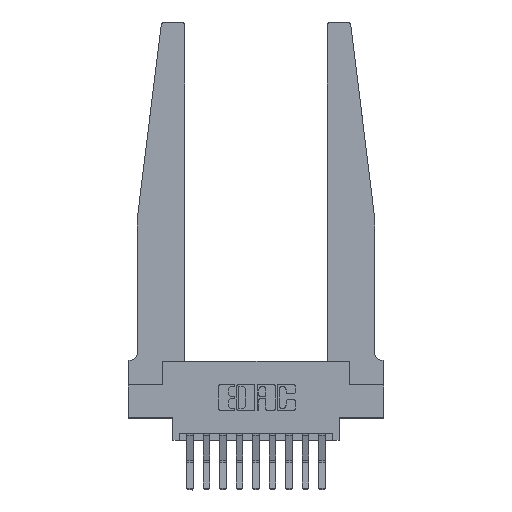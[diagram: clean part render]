
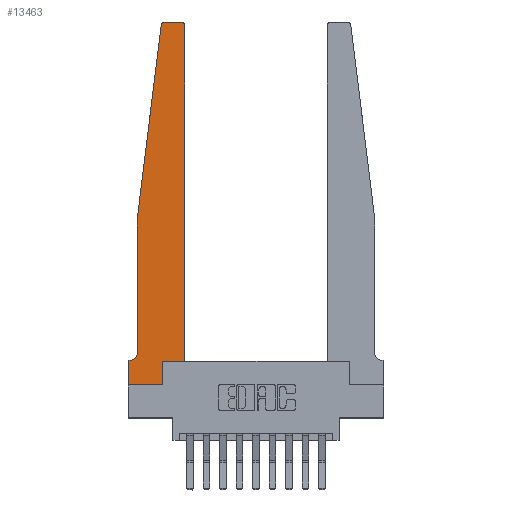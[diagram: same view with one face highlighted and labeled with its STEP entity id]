
A CAD part, top view. The second image highlights one B-rep face of the part: STEP entity #13463.
In plain terms, the highlighted planar face has unit normal (0, 0, 1).
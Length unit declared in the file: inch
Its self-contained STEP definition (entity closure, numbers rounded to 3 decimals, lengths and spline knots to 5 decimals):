
#108 = AXIS2_PLACEMENT_3D ( 'NONE', #7284, #8476, #1395 ) ;
#191 = ORIENTED_EDGE ( 'NONE', *, *, #7530, .T. ) ;
#193 = CARTESIAN_POINT ( 'NONE',  ( 0.2605, 0., 0.37 ) ) ;
#221 = VERTEX_POINT ( 'NONE', #193 ) ;
#870 = EDGE_CURVE ( 'NONE', #2707, #9263, #13168, .T. ) ;
#991 = VECTOR ( 'NONE', #13193, 39.37008 ) ;
#1066 = CARTESIAN_POINT ( 'NONE',  ( 0.395, 2.75, 0.37 ) ) ;
#1073 = LINE ( 'NONE', #15051, #13970 ) ;
#1248 = CARTESIAN_POINT ( 'NONE',  ( 0.2605, 0.18, 0.37 ) ) ;
#1303 = VERTEX_POINT ( 'NONE', #1066 ) ;
#1309 = EDGE_CURVE ( 'NONE', #4914, #3187, #11144, .T. ) ;
#1395 = DIRECTION ( 'NONE',  ( 1., 0., 0. ) ) ;
#1493 = CARTESIAN_POINT ( 'NONE',  ( 0.425, 0.18, 0.37 ) ) ;
#1557 = EDGE_CURVE ( 'NONE', #15088, #3222, #2284, .T. ) ;
#1620 = EDGE_CURVE ( 'NONE', #221, #3183, #10572, .T. ) ;
#1846 = DIRECTION ( 'NONE',  ( 1., 0., 0. ) ) ;
#2101 = CARTESIAN_POINT ( 'NONE',  ( 0., 0.1875, 0.37 ) ) ;
#2284 = LINE ( 'NONE', #1493, #11316 ) ;
#2380 = DIRECTION ( 'NONE',  ( 0., 0., 1. ) ) ;
#2623 = LINE ( 'NONE', #3178, #14767 ) ;
#2625 = VERTEX_POINT ( 'NONE', #4677 ) ;
#2666 = EDGE_CURVE ( 'NONE', #4063, #11071, #14952, .T. ) ;
#2689 = DIRECTION ( 'NONE',  ( 0., 1., 0. ) ) ;
#2707 = VERTEX_POINT ( 'NONE', #9500 ) ;
#2917 = EDGE_CURVE ( 'NONE', #3187, #4063, #2623, .T. ) ;
#3178 = CARTESIAN_POINT ( 'NONE',  ( 0.065, 0.1875, 0.37 ) ) ;
#3183 = VERTEX_POINT ( 'NONE', #1248 ) ;
#3187 = VERTEX_POINT ( 'NONE', #4842 ) ;
#3222 = VERTEX_POINT ( 'NONE', #7240 ) ;
#3589 = EDGE_CURVE ( 'NONE', #2625, #2707, #13636, .T. ) ;
#3675 = CARTESIAN_POINT ( 'NONE',  ( 0.065, 0.2375, 0.37 ) ) ;
#3740 = ORIENTED_EDGE ( 'NONE', *, *, #9920, .T. ) ;
#3920 = VECTOR ( 'NONE', #14111, 39.37008 ) ;
#4030 = CARTESIAN_POINT ( 'NONE',  ( 0.425, 0.18, 0.37 ) ) ;
#4063 = VERTEX_POINT ( 'NONE', #2101 ) ;
#4285 = ORIENTED_EDGE ( 'NONE', *, *, #3589, .T. ) ;
#4318 = VECTOR ( 'NONE', #8672, 39.37008 ) ;
#4478 = VECTOR ( 'NONE', #1846, 39.37008 ) ;
#4657 = CARTESIAN_POINT ( 'NONE',  ( 0.015, 0.2375, 0.37 ) ) ;
#4659 = EDGE_CURVE ( 'NONE', #1303, #2625, #1073, .T. ) ;
#4677 = CARTESIAN_POINT ( 'NONE',  ( 0.27653, 2.75, 0.37 ) ) ;
#4711 = DIRECTION ( 'NONE',  ( 0., 0., 1. ) ) ;
#4842 = CARTESIAN_POINT ( 'NONE',  ( 0.015, 0.1875, 0.37 ) ) ;
#4914 = VERTEX_POINT ( 'NONE', #3675 ) ;
#5268 = DIRECTION ( 'NONE',  ( 0., -1., 0. ) ) ;
#5409 = ORIENTED_EDGE ( 'NONE', *, *, #1557, .T. ) ;
#5853 = DIRECTION ( 'NONE',  ( -1., 0., 0. ) ) ;
#6107 = PLANE ( 'NONE',  #108 ) ;
#6480 = CIRCLE ( 'NONE', #12858, 0.03 ) ;
#6740 = DIRECTION ( 'NONE',  ( -1., 0., 0. ) ) ;
#6756 = EDGE_CURVE ( 'NONE', #3183, #15088, #8065, .T. ) ;
#7082 = CARTESIAN_POINT ( 'NONE',  ( 0., 0., 0.37 ) ) ;
#7240 = CARTESIAN_POINT ( 'NONE',  ( 0.425, 2.72, 0.37 ) ) ;
#7284 = CARTESIAN_POINT ( 'NONE',  ( 0., 0.1875, 0.37 ) ) ;
#7308 = CARTESIAN_POINT ( 'NONE',  ( 0., 0., 0.37 ) ) ;
#7530 = EDGE_CURVE ( 'NONE', #11071, #221, #8351, .T. ) ;
#7549 = DIRECTION ( 'NONE',  ( 1., 0., 0. ) ) ;
#7796 = ORIENTED_EDGE ( 'NONE', *, *, #14000, .T. ) ;
#8016 = DIRECTION ( 'NONE',  ( -1., 0., 0. ) ) ;
#8065 = LINE ( 'NONE', #13390, #13930 ) ;
#8351 = LINE ( 'NONE', #12380, #4478 ) ;
#8476 = DIRECTION ( 'NONE',  ( 0., 0., 1. ) ) ;
#8583 = CARTESIAN_POINT ( 'NONE',  ( 0.065, 1.25, 0.37 ) ) ;
#8672 = DIRECTION ( 'NONE',  ( 0., 1., 0. ) ) ;
#8943 = CARTESIAN_POINT ( 'NONE',  ( 0.065, 1.25, 0.37 ) ) ;
#9263 = VERTEX_POINT ( 'NONE', #8943 ) ;
#9265 = ORIENTED_EDGE ( 'NONE', *, *, #870, .T. ) ;
#9418 = CARTESIAN_POINT ( 'NONE',  ( 0.395, 2.72, 0.37 ) ) ;
#9457 = ORIENTED_EDGE ( 'NONE', *, *, #4659, .T. ) ;
#9500 = CARTESIAN_POINT ( 'NONE',  ( 0.24675, 2.72367, 0.37 ) ) ;
#9920 = EDGE_CURVE ( 'NONE', #3222, #1303, #6480, .T. ) ;
#10572 = LINE ( 'NONE', #14509, #4318 ) ;
#10616 = DIRECTION ( 'NONE',  ( 1., 0., 0. ) ) ;
#10920 = ORIENTED_EDGE ( 'NONE', *, *, #1309, .T. ) ;
#11071 = VERTEX_POINT ( 'NONE', #7308 ) ;
#11144 = CIRCLE ( 'NONE', #11884, 0.05 ) ;
#11279 = ORIENTED_EDGE ( 'NONE', *, *, #2666, .T. ) ;
#11301 = VECTOR ( 'NONE', #5268, 39.37008 ) ;
#11316 = VECTOR ( 'NONE', #2689, 39.37008 ) ;
#11429 = EDGE_LOOP ( 'NONE', ( #9457, #4285, #9265, #7796, #10920, #12386, #11279, #191, #14391, #12753, #5409, #3740 ) ) ;
#11738 = CARTESIAN_POINT ( 'NONE',  ( 0.27653, 2.72, 0.37 ) ) ;
#11884 = AXIS2_PLACEMENT_3D ( 'NONE', #4657, #12871, #5853 ) ;
#12230 = CARTESIAN_POINT ( 'NONE',  ( 0.065, 1.25, 0.37 ) ) ;
#12380 = CARTESIAN_POINT ( 'NONE',  ( 0., 0., 0.37 ) ) ;
#12386 = ORIENTED_EDGE ( 'NONE', *, *, #2917, .T. ) ;
#12405 = FACE_OUTER_BOUND ( 'NONE', #11429, .T. ) ;
#12753 = ORIENTED_EDGE ( 'NONE', *, *, #6756, .T. ) ;
#12858 = AXIS2_PLACEMENT_3D ( 'NONE', #9418, #2380, #10616 ) ;
#12871 = DIRECTION ( 'NONE',  ( 0., 0., -1. ) ) ;
#12924 = DIRECTION ( 'NONE',  ( 1., 0., 0. ) ) ;
#13168 = LINE ( 'NONE', #8583, #991 ) ;
#13193 = DIRECTION ( 'NONE',  ( -0.122, -0.992, 0. ) ) ;
#13390 = CARTESIAN_POINT ( 'NONE',  ( 0.425, 0.18, 0.37 ) ) ;
#13463 = ADVANCED_FACE ( 'NONE', ( #12405 ), #6107, .T. ) ;
#13636 = CIRCLE ( 'NONE', #13773, 0.03 ) ;
#13773 = AXIS2_PLACEMENT_3D ( 'NONE', #11738, #4711, #12924 ) ;
#13930 = VECTOR ( 'NONE', #7549, 39.37008 ) ;
#13970 = VECTOR ( 'NONE', #8016, 39.37008 ) ;
#14000 = EDGE_CURVE ( 'NONE', #9263, #4914, #15167, .T. ) ;
#14111 = DIRECTION ( 'NONE',  ( 0., -1., 0. ) ) ;
#14391 = ORIENTED_EDGE ( 'NONE', *, *, #1620, .T. ) ;
#14509 = CARTESIAN_POINT ( 'NONE',  ( 0.2605, 0.18, 0.37 ) ) ;
#14767 = VECTOR ( 'NONE', #6740, 39.37008 ) ;
#14952 = LINE ( 'NONE', #7082, #3920 ) ;
#15051 = CARTESIAN_POINT ( 'NONE',  ( 0.25, 2.75, 0.37 ) ) ;
#15088 = VERTEX_POINT ( 'NONE', #4030 ) ;
#15167 = LINE ( 'NONE', #12230, #11301 ) ;
